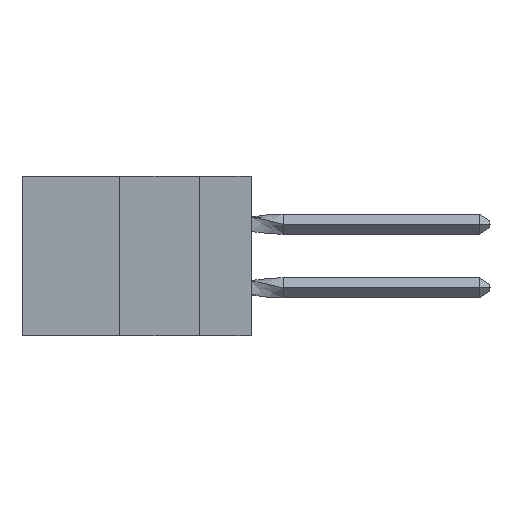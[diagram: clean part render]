
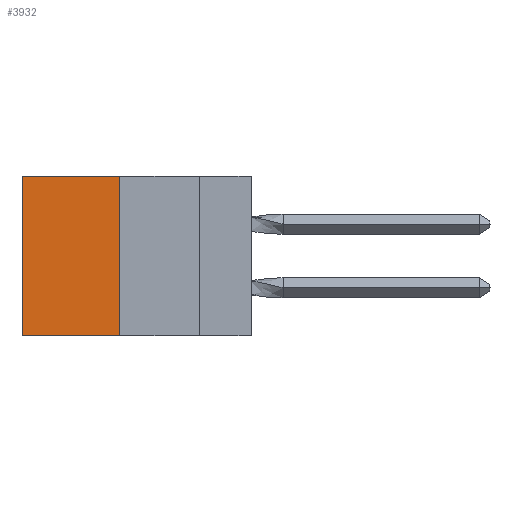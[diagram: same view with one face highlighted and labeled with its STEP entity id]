
A CAD part, left-side view. The second image highlights one B-rep face of the part: STEP entity #3932.
In plain terms, the highlighted planar face has unit normal (-1, 0, 0).
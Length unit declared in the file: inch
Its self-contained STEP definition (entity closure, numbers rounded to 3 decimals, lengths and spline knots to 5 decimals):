
#32 = DIRECTION ( 'NONE',  ( 1., 0., 0. ) ) ;
#1937 = CARTESIAN_POINT ( 'NONE',  ( 0.305, 0.413, -0.5 ) ) ;
#2074 = EDGE_LOOP ( 'NONE', ( #13669, #17989, #18251, #9032 ) ) ;
#2348 = LINE ( 'NONE', #14939, #3052 ) ;
#3052 = VECTOR ( 'NONE', #21506, 39.37008 ) ;
#3932 = ADVANCED_FACE ( 'NONE', ( #9943 ), #17181, .F. ) ;
#5089 = EDGE_CURVE ( 'NONE', #21484, #11842, #2348, .T. ) ;
#5482 = VECTOR ( 'NONE', #17402, 39.37008 ) ;
#7378 = DIRECTION ( 'NONE',  ( 0., 1., 0. ) ) ;
#7862 = CARTESIAN_POINT ( 'NONE',  ( 0.305, 0.413, 0. ) ) ;
#7948 = EDGE_CURVE ( 'NONE', #22427, #21484, #26296, .T. ) ;
#9032 = ORIENTED_EDGE ( 'NONE', *, *, #12194, .T. ) ;
#9603 = CARTESIAN_POINT ( 'NONE',  ( 0.305, 0.72, -0.5 ) ) ;
#9943 = FACE_OUTER_BOUND ( 'NONE', #2074, .T. ) ;
#10187 = CARTESIAN_POINT ( 'NONE',  ( 0.305, 0.413, 0. ) ) ;
#11842 = VERTEX_POINT ( 'NONE', #9603 ) ;
#12194 = EDGE_CURVE ( 'NONE', #22427, #14519, #22003, .T. ) ;
#12956 = DIRECTION ( 'NONE',  ( 0., 0., -1. ) ) ;
#13669 = ORIENTED_EDGE ( 'NONE', *, *, #19285, .T. ) ;
#14519 = VERTEX_POINT ( 'NONE', #19246 ) ;
#14939 = CARTESIAN_POINT ( 'NONE',  ( 0.305, 0.413, -0.5 ) ) ;
#16330 = VECTOR ( 'NONE', #27090, 39.37008 ) ;
#17181 = PLANE ( 'NONE',  #18144 ) ;
#17402 = DIRECTION ( 'NONE',  ( 0., 0., -1. ) ) ;
#17803 = CARTESIAN_POINT ( 'NONE',  ( 0.305, 0.413, -0.5 ) ) ;
#17989 = ORIENTED_EDGE ( 'NONE', *, *, #5089, .F. ) ;
#18144 = AXIS2_PLACEMENT_3D ( 'NONE', #1937, #32, #12956 ) ;
#18251 = ORIENTED_EDGE ( 'NONE', *, *, #7948, .F. ) ;
#19246 = CARTESIAN_POINT ( 'NONE',  ( 0.305, 0.72, 0. ) ) ;
#19285 = EDGE_CURVE ( 'NONE', #14519, #11842, #26246, .T. ) ;
#19567 = CARTESIAN_POINT ( 'NONE',  ( 0.305, 0.72, -0.5 ) ) ;
#21484 = VERTEX_POINT ( 'NONE', #17803 ) ;
#21506 = DIRECTION ( 'NONE',  ( 0., 1., 0. ) ) ;
#22003 = LINE ( 'NONE', #10187, #27107 ) ;
#22427 = VERTEX_POINT ( 'NONE', #7862 ) ;
#25989 = CARTESIAN_POINT ( 'NONE',  ( 0.305, 0.413, -0.5 ) ) ;
#26246 = LINE ( 'NONE', #19567, #16330 ) ;
#26296 = LINE ( 'NONE', #25989, #5482 ) ;
#27090 = DIRECTION ( 'NONE',  ( 0., 0., -1. ) ) ;
#27107 = VECTOR ( 'NONE', #7378, 39.37008 ) ;
